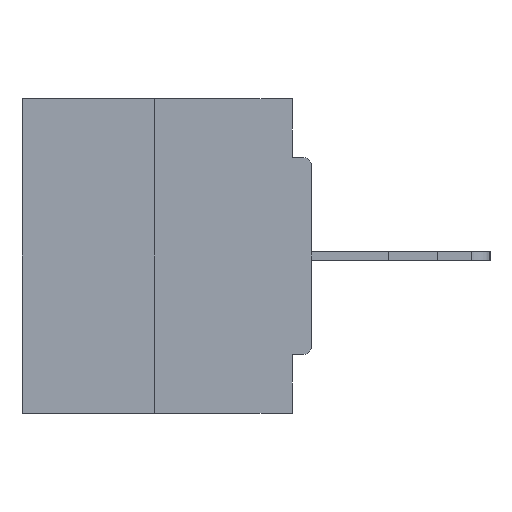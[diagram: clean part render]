
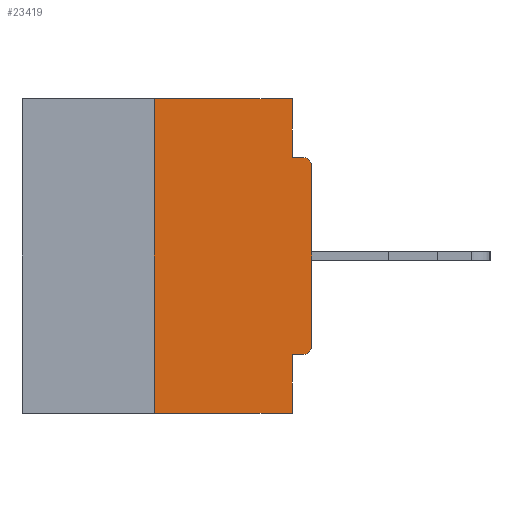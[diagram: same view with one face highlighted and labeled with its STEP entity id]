
A CAD part, left-side view. The second image highlights one B-rep face of the part: STEP entity #23419.
In plain terms, the highlighted planar face has unit normal (-1, 0, 0).
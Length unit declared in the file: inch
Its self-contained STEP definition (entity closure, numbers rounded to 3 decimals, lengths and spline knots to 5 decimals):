
#265 = LINE ( 'NONE', #4360, #21890 ) ;
#340 = CIRCLE ( 'NONE', #20339, 0.015 ) ;
#809 = AXIS2_PLACEMENT_3D ( 'NONE', #14788, #34034, #17611 ) ;
#1591 = VERTEX_POINT ( 'NONE', #9091 ) ;
#1635 = EDGE_CURVE ( 'NONE', #12010, #1591, #30099, .T. ) ;
#1937 = DIRECTION ( 'NONE',  ( 0., -1., 0. ) ) ;
#2901 = DIRECTION ( 'NONE',  ( 0., 0., 1. ) ) ;
#3182 = LINE ( 'NONE', #11272, #18242 ) ;
#4265 = CARTESIAN_POINT ( 'NONE',  ( 0., 0.031, -0.0935 ) ) ;
#4349 = LINE ( 'NONE', #19816, #34760 ) ;
#4360 = CARTESIAN_POINT ( 'NONE',  ( 0., 0., -0.4065 ) ) ;
#4951 = CARTESIAN_POINT ( 'NONE',  ( 0., 0.25, -0.5 ) ) ;
#6150 = DIRECTION ( 'NONE',  ( 0., -1., 0. ) ) ;
#6664 = EDGE_CURVE ( 'NONE', #30833, #14670, #18990, .T. ) ;
#7982 = VECTOR ( 'NONE', #14925, 39.37008 ) ;
#8444 = CARTESIAN_POINT ( 'NONE',  ( 0., 0.46, -0.5 ) ) ;
#8635 = EDGE_CURVE ( 'NONE', #29242, #27216, #265, .T. ) ;
#9091 = CARTESIAN_POINT ( 'NONE',  ( 0., 0.015, -0.0935 ) ) ;
#9980 = LINE ( 'NONE', #35290, #16565 ) ;
#10314 = PLANE ( 'NONE',  #34755 ) ;
#10992 = VECTOR ( 'NONE', #21778, 39.37008 ) ;
#11272 = CARTESIAN_POINT ( 'NONE',  ( 0., 0.031, 0. ) ) ;
#12010 = VERTEX_POINT ( 'NONE', #4265 ) ;
#12866 = VECTOR ( 'NONE', #35562, 39.37008 ) ;
#12879 = DIRECTION ( 'NONE',  ( 0., 1., 0. ) ) ;
#13784 = ORIENTED_EDGE ( 'NONE', *, *, #17821, .F. ) ;
#14000 = DIRECTION ( 'NONE',  ( -1., 0., 0. ) ) ;
#14067 = ORIENTED_EDGE ( 'NONE', *, *, #14195, .F. ) ;
#14195 = EDGE_CURVE ( 'NONE', #30833, #31336, #4349, .T. ) ;
#14214 = CIRCLE ( 'NONE', #809, 0.015 ) ;
#14670 = VERTEX_POINT ( 'NONE', #21736 ) ;
#14788 = CARTESIAN_POINT ( 'NONE',  ( 0., 0.015, -0.1085 ) ) ;
#14925 = DIRECTION ( 'NONE',  ( 0., -1., 0. ) ) ;
#15254 = ORIENTED_EDGE ( 'NONE', *, *, #6664, .T. ) ;
#15290 = ORIENTED_EDGE ( 'NONE', *, *, #29705, .F. ) ;
#16361 = CARTESIAN_POINT ( 'NONE',  ( 0., 0.031, -0.5 ) ) ;
#16565 = VECTOR ( 'NONE', #1937, 39.37008 ) ;
#16586 = ORIENTED_EDGE ( 'NONE', *, *, #8635, .F. ) ;
#16727 = CARTESIAN_POINT ( 'NONE',  ( 0., 0., -0.0935 ) ) ;
#16783 = CARTESIAN_POINT ( 'NONE',  ( 0., 0.015, -0.4065 ) ) ;
#17611 = DIRECTION ( 'NONE',  ( 0., 0., -1. ) ) ;
#17821 = EDGE_CURVE ( 'NONE', #31336, #18688, #9980, .T. ) ;
#18242 = VECTOR ( 'NONE', #33351, 39.37008 ) ;
#18450 = CARTESIAN_POINT ( 'NONE',  ( 0., 0.25, 0. ) ) ;
#18658 = EDGE_CURVE ( 'NONE', #18688, #12010, #3182, .T. ) ;
#18688 = VERTEX_POINT ( 'NONE', #28109 ) ;
#18738 = DIRECTION ( 'NONE',  ( 0., 0., -1. ) ) ;
#18990 = LINE ( 'NONE', #8444, #19852 ) ;
#19406 = EDGE_CURVE ( 'NONE', #19478, #1591, #14214, .T. ) ;
#19478 = VERTEX_POINT ( 'NONE', #28902 ) ;
#19816 = CARTESIAN_POINT ( 'NONE',  ( 0., 0.25, 0. ) ) ;
#19852 = VECTOR ( 'NONE', #6150, 39.37008 ) ;
#20064 = ORIENTED_EDGE ( 'NONE', *, *, #34093, .T. ) ;
#20339 = AXIS2_PLACEMENT_3D ( 'NONE', #30522, #14000, #33252 ) ;
#20527 = ORIENTED_EDGE ( 'NONE', *, *, #34559, .T. ) ;
#20902 = ORIENTED_EDGE ( 'NONE', *, *, #19406, .T. ) ;
#21215 = ORIENTED_EDGE ( 'NONE', *, *, #1635, .F. ) ;
#21284 = ORIENTED_EDGE ( 'NONE', *, *, #18658, .F. ) ;
#21736 = CARTESIAN_POINT ( 'NONE',  ( 0., 0.031, -0.5 ) ) ;
#21778 = DIRECTION ( 'NONE',  ( 0., 0., 1. ) ) ;
#21890 = VECTOR ( 'NONE', #12879, 39.37008 ) ;
#23419 = ADVANCED_FACE ( 'NONE', ( #30630 ), #10314, .F. ) ;
#25939 = LINE ( 'NONE', #16361, #12866 ) ;
#26816 = CARTESIAN_POINT ( 'NONE',  ( 0., 0.46, 0. ) ) ;
#27216 = VERTEX_POINT ( 'NONE', #32009 ) ;
#27281 = CARTESIAN_POINT ( 'NONE',  ( 0., 0., 0. ) ) ;
#27651 = CARTESIAN_POINT ( 'NONE',  ( 0., 0., -0.3915 ) ) ;
#28109 = CARTESIAN_POINT ( 'NONE',  ( 0., 0.031, 0. ) ) ;
#28902 = CARTESIAN_POINT ( 'NONE',  ( 0., 0., -0.1085 ) ) ;
#29242 = VERTEX_POINT ( 'NONE', #16783 ) ;
#29705 = EDGE_CURVE ( 'NONE', #27216, #14670, #25939, .T. ) ;
#30099 = LINE ( 'NONE', #16727, #7982 ) ;
#30522 = CARTESIAN_POINT ( 'NONE',  ( 0., 0.015, -0.3915 ) ) ;
#30630 = FACE_OUTER_BOUND ( 'NONE', #31008, .T. ) ;
#30833 = VERTEX_POINT ( 'NONE', #4951 ) ;
#31008 = EDGE_LOOP ( 'NONE', ( #13784, #14067, #15254, #15290, #16586, #20064, #20527, #20902, #21215, #21284 ) ) ;
#31336 = VERTEX_POINT ( 'NONE', #18450 ) ;
#32009 = CARTESIAN_POINT ( 'NONE',  ( 0., 0.031, -0.4065 ) ) ;
#32051 = VERTEX_POINT ( 'NONE', #27651 ) ;
#32992 = LINE ( 'NONE', #27281, #10992 ) ;
#33252 = DIRECTION ( 'NONE',  ( 0., 0., -1. ) ) ;
#33351 = DIRECTION ( 'NONE',  ( 0., 0., -1. ) ) ;
#34034 = DIRECTION ( 'NONE',  ( -1., 0., 0. ) ) ;
#34093 = EDGE_CURVE ( 'NONE', #29242, #32051, #340, .T. ) ;
#34559 = EDGE_CURVE ( 'NONE', #32051, #19478, #32992, .T. ) ;
#34755 = AXIS2_PLACEMENT_3D ( 'NONE', #26816, #35143, #18738 ) ;
#34760 = VECTOR ( 'NONE', #2901, 39.37008 ) ;
#35143 = DIRECTION ( 'NONE',  ( 1., 0., 0. ) ) ;
#35290 = CARTESIAN_POINT ( 'NONE',  ( 0., 0.46, 0. ) ) ;
#35562 = DIRECTION ( 'NONE',  ( 0., 0., -1. ) ) ;
